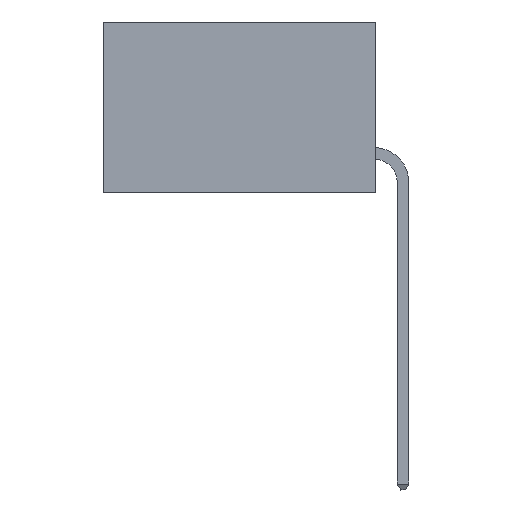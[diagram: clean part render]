
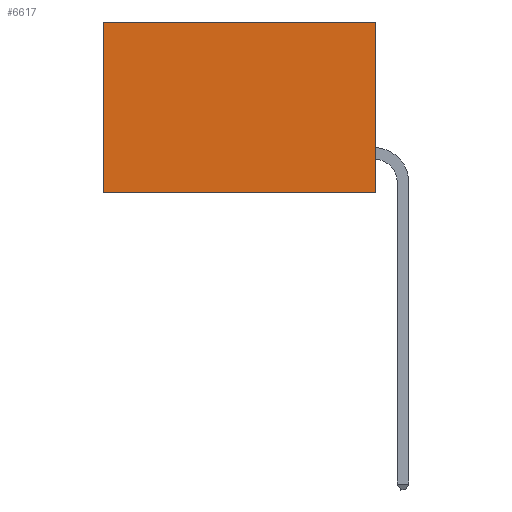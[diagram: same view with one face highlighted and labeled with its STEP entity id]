
A CAD part, left-side view. The second image highlights one B-rep face of the part: STEP entity #6617.
In plain terms, the highlighted planar face has unit normal (-1, 0, 0).
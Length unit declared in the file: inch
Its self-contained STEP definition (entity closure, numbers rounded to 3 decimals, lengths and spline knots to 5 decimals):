
#114 = EDGE_CURVE ( 'NONE', #12773, #7955, #10908, .T. ) ;
#594 = ORIENTED_EDGE ( 'NONE', *, *, #9916, .T. ) ;
#750 = CARTESIAN_POINT ( 'NONE',  ( 0.277, 0.59, -0.37 ) ) ;
#763 = ORIENTED_EDGE ( 'NONE', *, *, #9496, .F. ) ;
#1427 = ORIENTED_EDGE ( 'NONE', *, *, #114, .F. ) ;
#1584 = DIRECTION ( 'NONE',  ( 0., 0., -1. ) ) ;
#2256 = VECTOR ( 'NONE', #9645, 39.37008 ) ;
#2583 = LINE ( 'NONE', #5638, #2256 ) ;
#3037 = ORIENTED_EDGE ( 'NONE', *, *, #5194, .T. ) ;
#3169 = CARTESIAN_POINT ( 'NONE',  ( 0.277, 0., 0. ) ) ;
#3511 = VERTEX_POINT ( 'NONE', #750 ) ;
#3789 = VECTOR ( 'NONE', #7062, 39.37008 ) ;
#3898 = DIRECTION ( 'NONE',  ( 0., 0., -1. ) ) ;
#3910 = PLANE ( 'NONE',  #10382 ) ;
#3973 = CARTESIAN_POINT ( 'NONE',  ( 0.277, 0., -0.37 ) ) ;
#4129 = DIRECTION ( 'NONE',  ( 1., 0., 0. ) ) ;
#4475 = DIRECTION ( 'NONE',  ( 0., 0., -1. ) ) ;
#5124 = EDGE_LOOP ( 'NONE', ( #594, #763, #1427, #3037 ) ) ;
#5194 = EDGE_CURVE ( 'NONE', #12773, #7957, #12209, .T. ) ;
#5638 = CARTESIAN_POINT ( 'NONE',  ( 0.277, 0., -0.37 ) ) ;
#6157 = CARTESIAN_POINT ( 'NONE',  ( 0.277, 0., -0.37 ) ) ;
#6617 = ADVANCED_FACE ( 'NONE', ( #7886 ), #3910, .F. ) ;
#7062 = DIRECTION ( 'NONE',  ( 0., 1., 0. ) ) ;
#7173 = CARTESIAN_POINT ( 'NONE',  ( 0.277, 0., 0. ) ) ;
#7291 = CARTESIAN_POINT ( 'NONE',  ( 0.277, 0., -0.37 ) ) ;
#7886 = FACE_OUTER_BOUND ( 'NONE', #5124, .T. ) ;
#7955 = VERTEX_POINT ( 'NONE', #7291 ) ;
#7957 = VERTEX_POINT ( 'NONE', #9229 ) ;
#8411 = VECTOR ( 'NONE', #1584, 39.37008 ) ;
#9229 = CARTESIAN_POINT ( 'NONE',  ( 0.277, 0.59, 0. ) ) ;
#9496 = EDGE_CURVE ( 'NONE', #7955, #3511, #2583, .T. ) ;
#9645 = DIRECTION ( 'NONE',  ( 0., 1., 0. ) ) ;
#9876 = VECTOR ( 'NONE', #4475, 39.37008 ) ;
#9916 = EDGE_CURVE ( 'NONE', #7957, #3511, #12379, .T. ) ;
#10382 = AXIS2_PLACEMENT_3D ( 'NONE', #3973, #4129, #3898 ) ;
#10908 = LINE ( 'NONE', #6157, #8411 ) ;
#11317 = CARTESIAN_POINT ( 'NONE',  ( 0.277, 0.59, -0.37 ) ) ;
#12209 = LINE ( 'NONE', #7173, #3789 ) ;
#12379 = LINE ( 'NONE', #11317, #9876 ) ;
#12773 = VERTEX_POINT ( 'NONE', #3169 ) ;
